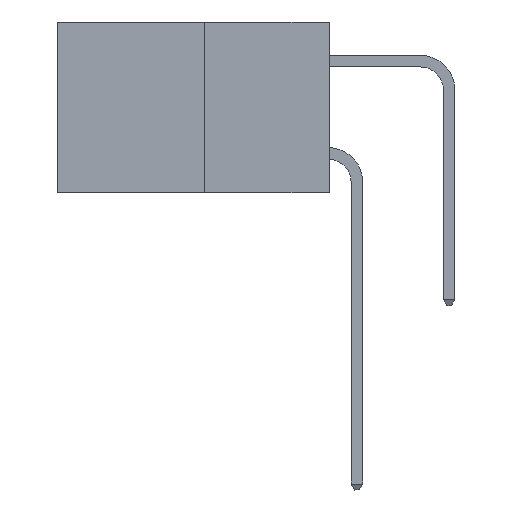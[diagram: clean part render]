
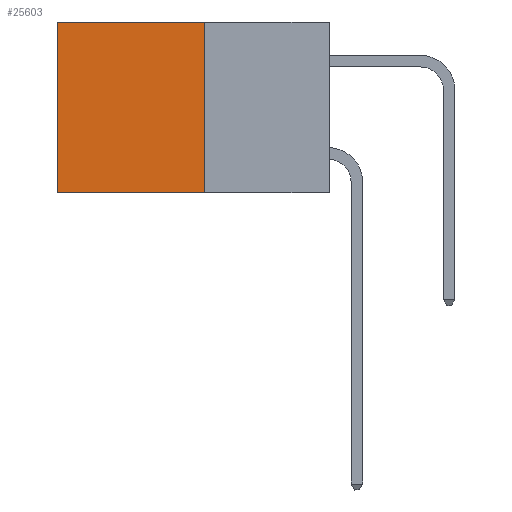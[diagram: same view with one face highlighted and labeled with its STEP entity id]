
A CAD part, left-side view. The second image highlights one B-rep face of the part: STEP entity #25603.
In plain terms, the highlighted planar face has unit normal (-1, 0, 0).
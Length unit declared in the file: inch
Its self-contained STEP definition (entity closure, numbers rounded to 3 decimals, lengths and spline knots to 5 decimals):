
#2043 = EDGE_CURVE ( 'NONE', #10908, #5819, #14661, .T. ) ;
#2453 = CARTESIAN_POINT ( 'NONE',  ( 0.277, 0.27, -0.37 ) ) ;
#2643 = CARTESIAN_POINT ( 'NONE',  ( 0.277, 0.59, -0.37 ) ) ;
#2848 = EDGE_CURVE ( 'NONE', #21769, #32349, #31324, .T. ) ;
#2983 = VECTOR ( 'NONE', #18519, 39.37008 ) ;
#3571 = ORIENTED_EDGE ( 'NONE', *, *, #2043, .F. ) ;
#3865 = LINE ( 'NONE', #2453, #2983 ) ;
#4653 = EDGE_CURVE ( 'NONE', #21769, #10908, #3865, .T. ) ;
#5639 = CARTESIAN_POINT ( 'NONE',  ( 0.277, 0.27, 0. ) ) ;
#5819 = VERTEX_POINT ( 'NONE', #2643 ) ;
#7529 = DIRECTION ( 'NONE',  ( 0., 1., 0. ) ) ;
#10145 = CARTESIAN_POINT ( 'NONE',  ( 0.277, 0.59, 0. ) ) ;
#10759 = CARTESIAN_POINT ( 'NONE',  ( 0.277, 0.27, 0. ) ) ;
#10908 = VERTEX_POINT ( 'NONE', #22998 ) ;
#12247 = DIRECTION ( 'NONE',  ( 0., 0., -1. ) ) ;
#12325 = ORIENTED_EDGE ( 'NONE', *, *, #4653, .F. ) ;
#14066 = DIRECTION ( 'NONE',  ( 1., 0., 0. ) ) ;
#14661 = LINE ( 'NONE', #21699, #35291 ) ;
#14819 = ORIENTED_EDGE ( 'NONE', *, *, #30231, .T. ) ;
#16928 = ORIENTED_EDGE ( 'NONE', *, *, #2848, .T. ) ;
#17264 = VECTOR ( 'NONE', #32136, 39.37008 ) ;
#18519 = DIRECTION ( 'NONE',  ( 0., 0., -1. ) ) ;
#20162 = AXIS2_PLACEMENT_3D ( 'NONE', #30936, #14066, #33728 ) ;
#21699 = CARTESIAN_POINT ( 'NONE',  ( 0.277, 0.27, -0.37 ) ) ;
#21769 = VERTEX_POINT ( 'NONE', #10759 ) ;
#22998 = CARTESIAN_POINT ( 'NONE',  ( 0.277, 0.27, -0.37 ) ) ;
#25217 = VECTOR ( 'NONE', #12247, 39.37008 ) ;
#25603 = ADVANCED_FACE ( 'NONE', ( #26020 ), #28156, .F. ) ;
#26020 = FACE_OUTER_BOUND ( 'NONE', #31216, .T. ) ;
#28156 = PLANE ( 'NONE',  #20162 ) ;
#30231 = EDGE_CURVE ( 'NONE', #32349, #5819, #32570, .T. ) ;
#30936 = CARTESIAN_POINT ( 'NONE',  ( 0.277, 0.27, -0.37 ) ) ;
#31216 = EDGE_LOOP ( 'NONE', ( #14819, #3571, #12325, #16928 ) ) ;
#31324 = LINE ( 'NONE', #5639, #17264 ) ;
#31957 = CARTESIAN_POINT ( 'NONE',  ( 0.277, 0.59, -0.37 ) ) ;
#32136 = DIRECTION ( 'NONE',  ( 0., 1., 0. ) ) ;
#32349 = VERTEX_POINT ( 'NONE', #10145 ) ;
#32570 = LINE ( 'NONE', #31957, #25217 ) ;
#33728 = DIRECTION ( 'NONE',  ( 0., 0., -1. ) ) ;
#35291 = VECTOR ( 'NONE', #7529, 39.37008 ) ;
